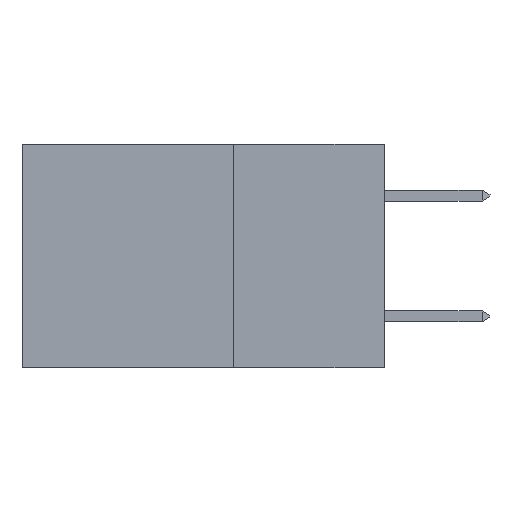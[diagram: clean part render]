
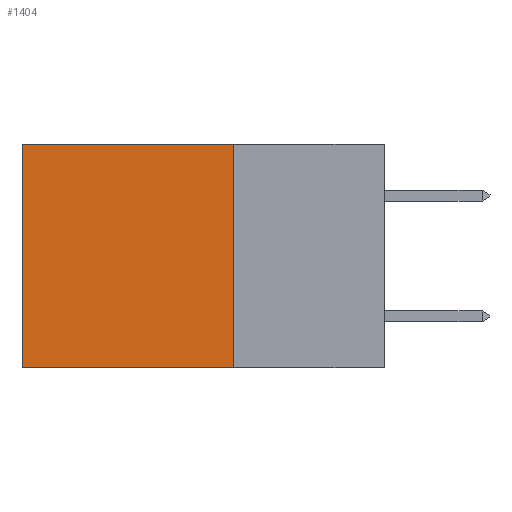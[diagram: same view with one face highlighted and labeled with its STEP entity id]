
A CAD part, left-side view. The second image highlights one B-rep face of the part: STEP entity #1404.
In plain terms, the highlighted planar face has unit normal (-1, 0, 0).
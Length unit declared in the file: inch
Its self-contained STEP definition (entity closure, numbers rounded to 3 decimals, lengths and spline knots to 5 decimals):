
#94 = DIRECTION ( 'NONE',  ( 1., 0., 0. ) ) ;
#1163 = VECTOR ( 'NONE', #14555, 39.37008 ) ;
#1251 = VECTOR ( 'NONE', #12913, 39.37008 ) ;
#1404 = ADVANCED_FACE ( 'NONE', ( #6601 ), #16097, .F. ) ;
#2433 = CARTESIAN_POINT ( 'NONE',  ( 0.2875, 0.25, -0.37 ) ) ;
#2806 = CARTESIAN_POINT ( 'NONE',  ( 0.2875, 0.6, -0.37 ) ) ;
#3065 = EDGE_CURVE ( 'NONE', #7620, #5739, #4883, .T. ) ;
#3196 = LINE ( 'NONE', #3461, #13921 ) ;
#3461 = CARTESIAN_POINT ( 'NONE',  ( 0.2875, 0.25, 0. ) ) ;
#3516 = LINE ( 'NONE', #15455, #16906 ) ;
#4808 = LINE ( 'NONE', #2433, #1163 ) ;
#4883 = LINE ( 'NONE', #8899, #1251 ) ;
#4934 = CARTESIAN_POINT ( 'NONE',  ( 0.2875, 0.25, 0. ) ) ;
#5192 = CARTESIAN_POINT ( 'NONE',  ( 0.2875, 0.25, 0. ) ) ;
#5304 = AXIS2_PLACEMENT_3D ( 'NONE', #4934, #94, #6843 ) ;
#5619 = VERTEX_POINT ( 'NONE', #5192 ) ;
#5739 = VERTEX_POINT ( 'NONE', #2806 ) ;
#6119 = DIRECTION ( 'NONE',  ( 0., 1., 0. ) ) ;
#6140 = DIRECTION ( 'NONE',  ( 0., 0., -1. ) ) ;
#6439 = ORIENTED_EDGE ( 'NONE', *, *, #3065, .T. ) ;
#6601 = FACE_OUTER_BOUND ( 'NONE', #12018, .T. ) ;
#6843 = DIRECTION ( 'NONE',  ( 0., 0., -1. ) ) ;
#6973 = ORIENTED_EDGE ( 'NONE', *, *, #13285, .F. ) ;
#7620 = VERTEX_POINT ( 'NONE', #10563 ) ;
#8173 = CARTESIAN_POINT ( 'NONE',  ( 0.2875, 0.25, -0.37 ) ) ;
#8899 = CARTESIAN_POINT ( 'NONE',  ( 0.2875, 0.6, 0. ) ) ;
#9414 = EDGE_CURVE ( 'NONE', #5619, #7620, #3516, .T. ) ;
#10052 = ORIENTED_EDGE ( 'NONE', *, *, #16838, .F. ) ;
#10563 = CARTESIAN_POINT ( 'NONE',  ( 0.2875, 0.6, 0. ) ) ;
#11892 = ORIENTED_EDGE ( 'NONE', *, *, #9414, .T. ) ;
#12018 = EDGE_LOOP ( 'NONE', ( #6439, #10052, #6973, #11892 ) ) ;
#12886 = VERTEX_POINT ( 'NONE', #8173 ) ;
#12913 = DIRECTION ( 'NONE',  ( 0., 0., -1. ) ) ;
#13285 = EDGE_CURVE ( 'NONE', #5619, #12886, #3196, .T. ) ;
#13921 = VECTOR ( 'NONE', #6140, 39.37008 ) ;
#14555 = DIRECTION ( 'NONE',  ( 0., 1., 0. ) ) ;
#15455 = CARTESIAN_POINT ( 'NONE',  ( 0.2875, 0.25, 0. ) ) ;
#16097 = PLANE ( 'NONE',  #5304 ) ;
#16838 = EDGE_CURVE ( 'NONE', #12886, #5739, #4808, .T. ) ;
#16906 = VECTOR ( 'NONE', #6119, 39.37008 ) ;
